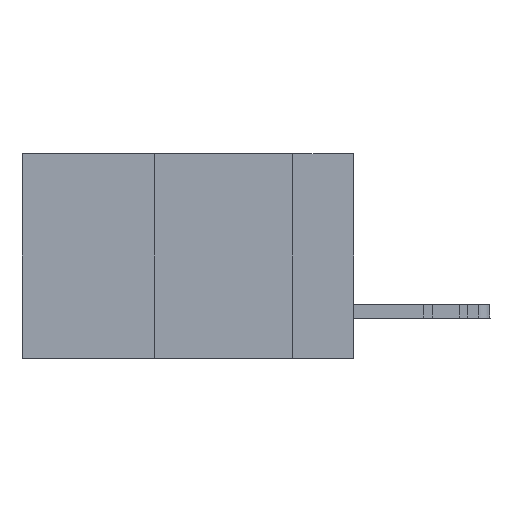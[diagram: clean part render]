
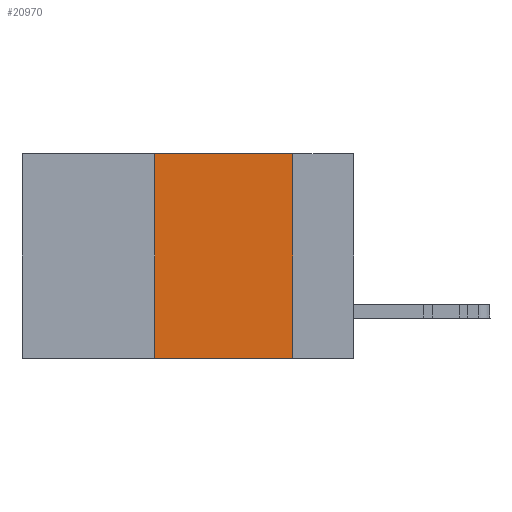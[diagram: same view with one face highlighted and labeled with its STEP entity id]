
A CAD part, left-side view. The second image highlights one B-rep face of the part: STEP entity #20970.
In plain terms, the highlighted planar face has unit normal (-1, 0, 0).
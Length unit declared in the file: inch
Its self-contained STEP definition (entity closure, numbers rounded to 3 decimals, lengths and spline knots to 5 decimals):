
#1827 = EDGE_LOOP ( 'NONE', ( #30224, #10096, #13440, #12095 ) ) ;
#3508 = VERTEX_POINT ( 'NONE', #38467 ) ;
#3667 = AXIS2_PLACEMENT_3D ( 'NONE', #14976, #4435, #7518 ) ;
#4435 = DIRECTION ( 'NONE',  ( 1., 0., 0. ) ) ;
#5938 = LINE ( 'NONE', #17411, #13602 ) ;
#7349 = LINE ( 'NONE', #37039, #11170 ) ;
#7518 = DIRECTION ( 'NONE',  ( 0., 0., -1. ) ) ;
#8115 = VECTOR ( 'NONE', #37613, 39.37008 ) ;
#10096 = ORIENTED_EDGE ( 'NONE', *, *, #27946, .F. ) ;
#10315 = DIRECTION ( 'NONE',  ( 0., 0., -1. ) ) ;
#11170 = VECTOR ( 'NONE', #26334, 39.37008 ) ;
#11313 = DIRECTION ( 'NONE',  ( 0., 0., 1. ) ) ;
#12095 = ORIENTED_EDGE ( 'NONE', *, *, #20982, .T. ) ;
#13440 = ORIENTED_EDGE ( 'NONE', *, *, #37754, .F. ) ;
#13602 = VECTOR ( 'NONE', #10315, 39.37008 ) ;
#14976 = CARTESIAN_POINT ( 'NONE',  ( 0., 0.6, 0. ) ) ;
#16092 = FACE_OUTER_BOUND ( 'NONE', #1827, .T. ) ;
#17411 = CARTESIAN_POINT ( 'NONE',  ( 0., 0.11, 0. ) ) ;
#20970 = ADVANCED_FACE ( 'NONE', ( #16092 ), #21325, .F. ) ;
#20982 = EDGE_CURVE ( 'NONE', #39542, #3508, #7349, .T. ) ;
#21325 = PLANE ( 'NONE',  #3667 ) ;
#26334 = DIRECTION ( 'NONE',  ( 0., -1., 0. ) ) ;
#27946 = EDGE_CURVE ( 'NONE', #28306, #30002, #42016, .T. ) ;
#28151 = EDGE_CURVE ( 'NONE', #30002, #3508, #5938, .T. ) ;
#28306 = VERTEX_POINT ( 'NONE', #39282 ) ;
#30002 = VERTEX_POINT ( 'NONE', #30737 ) ;
#30224 = ORIENTED_EDGE ( 'NONE', *, *, #28151, .F. ) ;
#30572 = CARTESIAN_POINT ( 'NONE',  ( 0., 0.6, 0. ) ) ;
#30737 = CARTESIAN_POINT ( 'NONE',  ( 0., 0.11, 0. ) ) ;
#34929 = LINE ( 'NONE', #39238, #36044 ) ;
#36044 = VECTOR ( 'NONE', #11313, 39.37008 ) ;
#37039 = CARTESIAN_POINT ( 'NONE',  ( 0., 0.6, -0.37 ) ) ;
#37613 = DIRECTION ( 'NONE',  ( 0., -1., 0. ) ) ;
#37754 = EDGE_CURVE ( 'NONE', #39542, #28306, #34929, .T. ) ;
#38467 = CARTESIAN_POINT ( 'NONE',  ( 0., 0.11, -0.37 ) ) ;
#39238 = CARTESIAN_POINT ( 'NONE',  ( 0., 0.36, 0. ) ) ;
#39282 = CARTESIAN_POINT ( 'NONE',  ( 0., 0.36, 0. ) ) ;
#39542 = VERTEX_POINT ( 'NONE', #42413 ) ;
#42016 = LINE ( 'NONE', #30572, #8115 ) ;
#42413 = CARTESIAN_POINT ( 'NONE',  ( 0., 0.36, -0.37 ) ) ;
